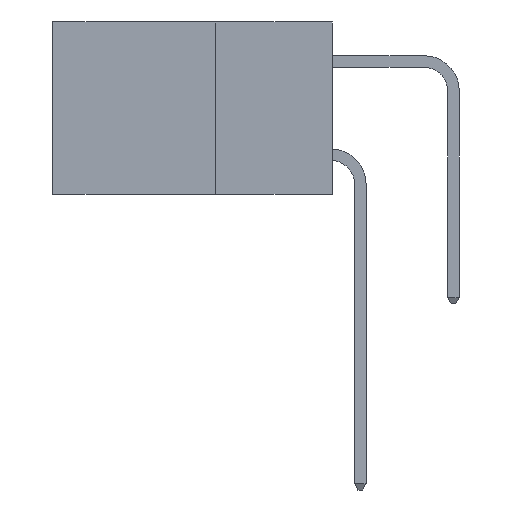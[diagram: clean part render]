
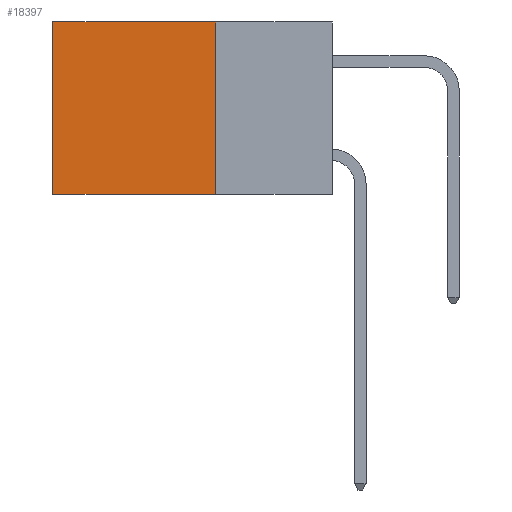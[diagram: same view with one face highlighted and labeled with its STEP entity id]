
A CAD part, left-side view. The second image highlights one B-rep face of the part: STEP entity #18397.
In plain terms, the highlighted planar face has unit normal (-1, 0, 0).
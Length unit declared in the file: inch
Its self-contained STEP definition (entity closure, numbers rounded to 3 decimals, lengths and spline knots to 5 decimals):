
#336 = ORIENTED_EDGE ( 'NONE', *, *, #28494, .T. ) ;
#1729 = ORIENTED_EDGE ( 'NONE', *, *, #2191, .F. ) ;
#2093 = DIRECTION ( 'NONE',  ( 0., 1., 0. ) ) ;
#2191 = EDGE_CURVE ( 'NONE', #18289, #14433, #19622, .T. ) ;
#3186 = VECTOR ( 'NONE', #6129, 39.37008 ) ;
#4634 = CARTESIAN_POINT ( 'NONE',  ( 0.2615, 0.25, 0. ) ) ;
#6129 = DIRECTION ( 'NONE',  ( 0., 0., -1. ) ) ;
#7238 = VECTOR ( 'NONE', #16863, 39.37008 ) ;
#8626 = VERTEX_POINT ( 'NONE', #24550 ) ;
#9540 = DIRECTION ( 'NONE',  ( 1., 0., 0. ) ) ;
#11850 = ORIENTED_EDGE ( 'NONE', *, *, #21727, .F. ) ;
#12376 = CARTESIAN_POINT ( 'NONE',  ( 0.2615, 0.25, 0. ) ) ;
#13428 = ORIENTED_EDGE ( 'NONE', *, *, #13431, .T. ) ;
#13431 = EDGE_CURVE ( 'NONE', #8626, #16120, #21842, .T. ) ;
#13446 = CARTESIAN_POINT ( 'NONE',  ( 0.2615, 0.25, -0.37 ) ) ;
#14433 = VERTEX_POINT ( 'NONE', #23325 ) ;
#15164 = EDGE_LOOP ( 'NONE', ( #13428, #11850, #1729, #336 ) ) ;
#15732 = AXIS2_PLACEMENT_3D ( 'NONE', #16240, #9540, #25126 ) ;
#16120 = VERTEX_POINT ( 'NONE', #19434 ) ;
#16240 = CARTESIAN_POINT ( 'NONE',  ( 0.2615, 0.25, -0.37 ) ) ;
#16863 = DIRECTION ( 'NONE',  ( 0., 1., 0. ) ) ;
#18289 = VERTEX_POINT ( 'NONE', #4634 ) ;
#18397 = ADVANCED_FACE ( 'NONE', ( #22039 ), #20693, .F. ) ;
#18514 = LINE ( 'NONE', #12376, #7238 ) ;
#18924 = VECTOR ( 'NONE', #22715, 39.37008 ) ;
#19434 = CARTESIAN_POINT ( 'NONE',  ( 0.2615, 0.6, -0.37 ) ) ;
#19622 = LINE ( 'NONE', #20523, #18924 ) ;
#20523 = CARTESIAN_POINT ( 'NONE',  ( 0.2615, 0.25, -0.37 ) ) ;
#20693 = PLANE ( 'NONE',  #15732 ) ;
#21727 = EDGE_CURVE ( 'NONE', #14433, #16120, #22572, .T. ) ;
#21825 = CARTESIAN_POINT ( 'NONE',  ( 0.2615, 0.6, -0.37 ) ) ;
#21842 = LINE ( 'NONE', #21825, #3186 ) ;
#22039 = FACE_OUTER_BOUND ( 'NONE', #15164, .T. ) ;
#22572 = LINE ( 'NONE', #13446, #27734 ) ;
#22715 = DIRECTION ( 'NONE',  ( 0., 0., -1. ) ) ;
#23325 = CARTESIAN_POINT ( 'NONE',  ( 0.2615, 0.25, -0.37 ) ) ;
#24550 = CARTESIAN_POINT ( 'NONE',  ( 0.2615, 0.6, 0. ) ) ;
#25126 = DIRECTION ( 'NONE',  ( 0., 0., -1. ) ) ;
#27734 = VECTOR ( 'NONE', #2093, 39.37008 ) ;
#28494 = EDGE_CURVE ( 'NONE', #18289, #8626, #18514, .T. ) ;
